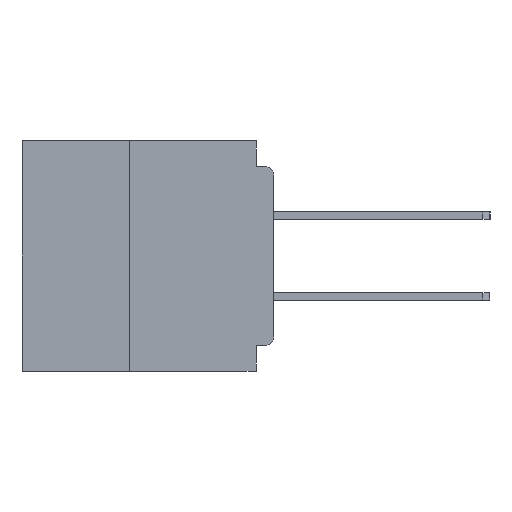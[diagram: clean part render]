
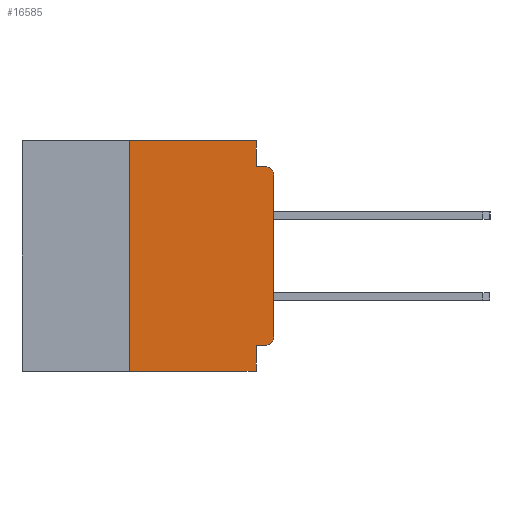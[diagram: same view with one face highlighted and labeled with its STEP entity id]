
A CAD part, left-side view. The second image highlights one B-rep face of the part: STEP entity #16585.
In plain terms, the highlighted planar face has unit normal (-1, 0, 0).
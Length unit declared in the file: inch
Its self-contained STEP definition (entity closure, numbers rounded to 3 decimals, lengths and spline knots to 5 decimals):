
#899 = CARTESIAN_POINT ( 'NONE',  ( 0., 0., 0. ) ) ;
#1323 = VERTEX_POINT ( 'NONE', #59244 ) ;
#1365 = VERTEX_POINT ( 'NONE', #57537 ) ;
#1514 = VERTEX_POINT ( 'NONE', #53215 ) ;
#2800 = CIRCLE ( 'NONE', #56232, 0.015 ) ;
#5500 = CARTESIAN_POINT ( 'NONE',  ( 0., 0.031, -0.4 ) ) ;
#6121 = DIRECTION ( 'NONE',  ( 0., -1., 0. ) ) ;
#6352 = FACE_OUTER_BOUND ( 'NONE', #30504, .T. ) ;
#7540 = LINE ( 'NONE', #42220, #42850 ) ;
#8280 = LINE ( 'NONE', #17450, #55721 ) ;
#9219 = DIRECTION ( 'NONE',  ( 0., 1., 0. ) ) ;
#9998 = EDGE_CURVE ( 'NONE', #15097, #1514, #7540, .T. ) ;
#10016 = CARTESIAN_POINT ( 'NONE',  ( 0., 0.015, -0.06 ) ) ;
#10176 = DIRECTION ( 'NONE',  ( 0., 0., 1. ) ) ;
#11221 = ORIENTED_EDGE ( 'NONE', *, *, #34019, .T. ) ;
#12454 = PLANE ( 'NONE',  #38289 ) ;
#14283 = ORIENTED_EDGE ( 'NONE', *, *, #25202, .F. ) ;
#14716 = DIRECTION ( 'NONE',  ( 0., 0., -1. ) ) ;
#15097 = VERTEX_POINT ( 'NONE', #23731 ) ;
#15272 = CARTESIAN_POINT ( 'NONE',  ( 0., 0., -0.045 ) ) ;
#16585 = ADVANCED_FACE ( 'NONE', ( #6352 ), #12454, .F. ) ;
#17450 = CARTESIAN_POINT ( 'NONE',  ( 0., 0.437, -0.4 ) ) ;
#17762 = CIRCLE ( 'NONE', #51323, 0.015 ) ;
#19115 = VECTOR ( 'NONE', #9219, 39.37008 ) ;
#19374 = DIRECTION ( 'NONE',  ( 0., 0., 1. ) ) ;
#20045 = CARTESIAN_POINT ( 'NONE',  ( 0., 0., -0.34 ) ) ;
#20064 = VERTEX_POINT ( 'NONE', #35051 ) ;
#20985 = CARTESIAN_POINT ( 'NONE',  ( 0., 0.031, -0.045 ) ) ;
#21084 = LINE ( 'NONE', #899, #53289 ) ;
#21726 = VECTOR ( 'NONE', #57032, 39.37008 ) ;
#21773 = DIRECTION ( 'NONE',  ( 1., 0., 0. ) ) ;
#22182 = VERTEX_POINT ( 'NONE', #20985 ) ;
#23162 = LINE ( 'NONE', #52428, #21726 ) ;
#23662 = CARTESIAN_POINT ( 'NONE',  ( 0., 0.015, -0.34 ) ) ;
#23731 = CARTESIAN_POINT ( 'NONE',  ( 0., 0.25, -0.4 ) ) ;
#24359 = ORIENTED_EDGE ( 'NONE', *, *, #58874, .F. ) ;
#24876 = ORIENTED_EDGE ( 'NONE', *, *, #31120, .F. ) ;
#24978 = DIRECTION ( 'NONE',  ( 0., -1., 0. ) ) ;
#25030 = ORIENTED_EDGE ( 'NONE', *, *, #9998, .F. ) ;
#25141 = VECTOR ( 'NONE', #24978, 39.37008 ) ;
#25202 = EDGE_CURVE ( 'NONE', #1514, #47145, #38743, .T. ) ;
#26677 = DIRECTION ( 'NONE',  ( 0., -1., 0. ) ) ;
#26704 = LINE ( 'NONE', #15272, #49629 ) ;
#26777 = DIRECTION ( 'NONE',  ( 0., 0., -1. ) ) ;
#28035 = ORIENTED_EDGE ( 'NONE', *, *, #29567, .F. ) ;
#28257 = DIRECTION ( 'NONE',  ( 0., 0., -1. ) ) ;
#29567 = EDGE_CURVE ( 'NONE', #1323, #33656, #44757, .T. ) ;
#29579 = CARTESIAN_POINT ( 'NONE',  ( 0., 0.437, 0. ) ) ;
#29851 = EDGE_CURVE ( 'NONE', #42213, #49179, #21084, .T. ) ;
#30504 = EDGE_LOOP ( 'NONE', ( #54150, #31313, #24359, #24876, #14283, #25030, #11221, #28035, #37412, #45838 ) ) ;
#31120 = EDGE_CURVE ( 'NONE', #47145, #22182, #23162, .T. ) ;
#31313 = ORIENTED_EDGE ( 'NONE', *, *, #56619, .T. ) ;
#33656 = VERTEX_POINT ( 'NONE', #5500 ) ;
#33979 = VECTOR ( 'NONE', #26777, 39.37008 ) ;
#34019 = EDGE_CURVE ( 'NONE', #15097, #33656, #8280, .T. ) ;
#34151 = LINE ( 'NONE', #55041, #19115 ) ;
#35051 = CARTESIAN_POINT ( 'NONE',  ( 0., 0.015, -0.045 ) ) ;
#35842 = CARTESIAN_POINT ( 'NONE',  ( 0., 0., -0.06 ) ) ;
#37412 = ORIENTED_EDGE ( 'NONE', *, *, #47552, .F. ) ;
#38289 = AXIS2_PLACEMENT_3D ( 'NONE', #44402, #21773, #53812 ) ;
#38668 = CARTESIAN_POINT ( 'NONE',  ( 0., 0.031, 0. ) ) ;
#38743 = LINE ( 'NONE', #29579, #25141 ) ;
#42213 = VERTEX_POINT ( 'NONE', #20045 ) ;
#42220 = CARTESIAN_POINT ( 'NONE',  ( 0., 0.25, -0.4 ) ) ;
#42228 = DIRECTION ( 'NONE',  ( -1., 0., 0. ) ) ;
#42850 = VECTOR ( 'NONE', #19374, 39.37008 ) ;
#44402 = CARTESIAN_POINT ( 'NONE',  ( 0., 0.437, 0. ) ) ;
#44757 = LINE ( 'NONE', #54213, #33979 ) ;
#45838 = ORIENTED_EDGE ( 'NONE', *, *, #54618, .T. ) ;
#47145 = VERTEX_POINT ( 'NONE', #38668 ) ;
#47552 = EDGE_CURVE ( 'NONE', #1365, #1323, #34151, .T. ) ;
#49179 = VERTEX_POINT ( 'NONE', #35842 ) ;
#49629 = VECTOR ( 'NONE', #6121, 39.37008 ) ;
#51323 = AXIS2_PLACEMENT_3D ( 'NONE', #10016, #42228, #14716 ) ;
#52428 = CARTESIAN_POINT ( 'NONE',  ( 0., 0.031, 0. ) ) ;
#53215 = CARTESIAN_POINT ( 'NONE',  ( 0., 0.25, 0. ) ) ;
#53289 = VECTOR ( 'NONE', #10176, 39.37008 ) ;
#53812 = DIRECTION ( 'NONE',  ( 0., 0., -1. ) ) ;
#54150 = ORIENTED_EDGE ( 'NONE', *, *, #29851, .T. ) ;
#54213 = CARTESIAN_POINT ( 'NONE',  ( 0., 0.031, -0.4 ) ) ;
#54618 = EDGE_CURVE ( 'NONE', #1365, #42213, #2800, .T. ) ;
#55041 = CARTESIAN_POINT ( 'NONE',  ( 0., 0., -0.355 ) ) ;
#55673 = DIRECTION ( 'NONE',  ( -1., 0., 0. ) ) ;
#55721 = VECTOR ( 'NONE', #26677, 39.37008 ) ;
#56232 = AXIS2_PLACEMENT_3D ( 'NONE', #23662, #55673, #28257 ) ;
#56619 = EDGE_CURVE ( 'NONE', #49179, #20064, #17762, .T. ) ;
#57032 = DIRECTION ( 'NONE',  ( 0., 0., -1. ) ) ;
#57537 = CARTESIAN_POINT ( 'NONE',  ( 0., 0.015, -0.355 ) ) ;
#58874 = EDGE_CURVE ( 'NONE', #22182, #20064, #26704, .T. ) ;
#59244 = CARTESIAN_POINT ( 'NONE',  ( 0., 0.031, -0.355 ) ) ;
